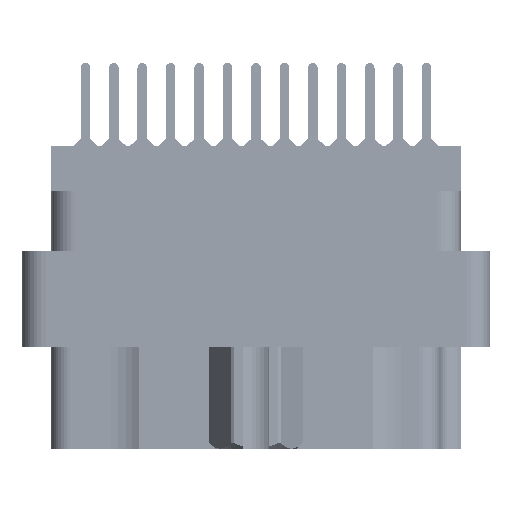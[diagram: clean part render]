
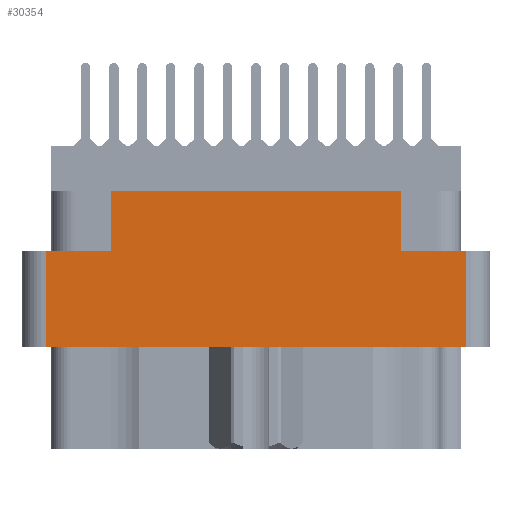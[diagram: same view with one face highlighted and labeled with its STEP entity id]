
A CAD part, left-side view. The second image highlights one B-rep face of the part: STEP entity #30354.
In plain terms, the highlighted planar face has unit normal (-1, 0, 0).
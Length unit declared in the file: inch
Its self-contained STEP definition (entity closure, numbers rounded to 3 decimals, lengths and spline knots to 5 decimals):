
#2329 = DIRECTION ( 'NONE',  ( 0., 1., 0. ) ) ;
#4207 = EDGE_LOOP ( 'NONE', ( #23088, #5940, #24946, #58882, #9343, #20774, #22834, #62159 ) ) ;
#4234 = EDGE_CURVE ( 'NONE', #32977, #33149, #74089, .T. ) ;
#4402 = VECTOR ( 'NONE', #29877, 39.37008 ) ;
#5191 = EDGE_CURVE ( 'NONE', #11066, #46096, #27409, .T. ) ;
#5940 = ORIENTED_EDGE ( 'NONE', *, *, #13438, .T. ) ;
#7363 = CARTESIAN_POINT ( 'NONE',  ( -1.359, 0.555, -0.798 ) ) ;
#7445 = AXIS2_PLACEMENT_3D ( 'NONE', #15939, #22190, #61098 ) ;
#8435 = CARTESIAN_POINT ( 'NONE',  ( -1.359, -0.555, -0.529 ) ) ;
#9343 = ORIENTED_EDGE ( 'NONE', *, *, #72518, .F. ) ;
#11066 = VERTEX_POINT ( 'NONE', #36326 ) ;
#12417 = CARTESIAN_POINT ( 'NONE',  ( -1.359, -0.555, -0.277 ) ) ;
#13404 = CARTESIAN_POINT ( 'NONE',  ( -1.359, 0.3825, -0.277 ) ) ;
#13438 = EDGE_CURVE ( 'NONE', #58204, #33149, #72020, .T. ) ;
#15939 = CARTESIAN_POINT ( 'NONE',  ( -1.359, -0.617, -0.798 ) ) ;
#17860 = DIRECTION ( 'NONE',  ( 0., 0., 1. ) ) ;
#20774 = ORIENTED_EDGE ( 'NONE', *, *, #37668, .T. ) ;
#22190 = DIRECTION ( 'NONE',  ( -1., 0., 0. ) ) ;
#22834 = ORIENTED_EDGE ( 'NONE', *, *, #73538, .F. ) ;
#23088 = ORIENTED_EDGE ( 'NONE', *, *, #38173, .F. ) ;
#23297 = PLANE ( 'NONE',  #7445 ) ;
#24946 = ORIENTED_EDGE ( 'NONE', *, *, #4234, .F. ) ;
#25122 = VERTEX_POINT ( 'NONE', #71787 ) ;
#27409 = LINE ( 'NONE', #13404, #76890 ) ;
#27895 = DIRECTION ( 'NONE',  ( 0., -1., 0. ) ) ;
#29877 = DIRECTION ( 'NONE',  ( 0., -1., 0. ) ) ;
#30354 = ADVANCED_FACE ( 'NONE', ( #48318 ), #23297, .T. ) ;
#30943 = VERTEX_POINT ( 'NONE', #12417 ) ;
#32977 = VERTEX_POINT ( 'NONE', #8435 ) ;
#33024 = CARTESIAN_POINT ( 'NONE',  ( -1.359, 0., -0.277 ) ) ;
#33149 = VERTEX_POINT ( 'NONE', #68557 ) ;
#36326 = CARTESIAN_POINT ( 'NONE',  ( -1.359, 0.3825, -0.277 ) ) ;
#36775 = VECTOR ( 'NONE', #70302, 39.37008 ) ;
#37668 = EDGE_CURVE ( 'NONE', #46288, #25122, #63082, .T. ) ;
#38173 = EDGE_CURVE ( 'NONE', #58204, #11066, #78127, .T. ) ;
#38374 = CARTESIAN_POINT ( 'NONE',  ( -1.359, 0.617, -0.117 ) ) ;
#39466 = CARTESIAN_POINT ( 'NONE',  ( -1.359, 0.555, -0.277 ) ) ;
#39832 = LINE ( 'NONE', #33024, #76165 ) ;
#41041 = CARTESIAN_POINT ( 'NONE',  ( -1.359, 0., -0.529 ) ) ;
#41786 = CARTESIAN_POINT ( 'NONE',  ( -1.359, 0., -0.277 ) ) ;
#46096 = VERTEX_POINT ( 'NONE', #60610 ) ;
#46288 = VERTEX_POINT ( 'NONE', #75838 ) ;
#46964 = DIRECTION ( 'NONE',  ( 0., 0., 1. ) ) ;
#47812 = LINE ( 'NONE', #38374, #36775 ) ;
#48318 = FACE_OUTER_BOUND ( 'NONE', #4207, .T. ) ;
#50732 = VECTOR ( 'NONE', #77898, 39.37008 ) ;
#53866 = VECTOR ( 'NONE', #2329, 39.37008 ) ;
#55731 = LINE ( 'NONE', #73322, #68923 ) ;
#57012 = VECTOR ( 'NONE', #17860, 39.37008 ) ;
#58204 = VERTEX_POINT ( 'NONE', #39466 ) ;
#58272 = EDGE_CURVE ( 'NONE', #32977, #30943, #55731, .T. ) ;
#58882 = ORIENTED_EDGE ( 'NONE', *, *, #58272, .T. ) ;
#60610 = CARTESIAN_POINT ( 'NONE',  ( -1.359, 0.3825, -0.117 ) ) ;
#61098 = DIRECTION ( 'NONE',  ( 0., 0., 1. ) ) ;
#62159 = ORIENTED_EDGE ( 'NONE', *, *, #5191, .F. ) ;
#63082 = LINE ( 'NONE', #68984, #57012 ) ;
#68557 = CARTESIAN_POINT ( 'NONE',  ( -1.359, 0.555, -0.529 ) ) ;
#68923 = VECTOR ( 'NONE', #78933, 39.37008 ) ;
#68984 = CARTESIAN_POINT ( 'NONE',  ( -1.359, -0.3825, -0.277 ) ) ;
#70302 = DIRECTION ( 'NONE',  ( 0., -1., 0. ) ) ;
#71787 = CARTESIAN_POINT ( 'NONE',  ( -1.359, -0.3825, -0.117 ) ) ;
#72020 = LINE ( 'NONE', #7363, #50732 ) ;
#72518 = EDGE_CURVE ( 'NONE', #46288, #30943, #39832, .T. ) ;
#73322 = CARTESIAN_POINT ( 'NONE',  ( -1.359, -0.555, -0.798 ) ) ;
#73538 = EDGE_CURVE ( 'NONE', #46096, #25122, #47812, .T. ) ;
#74089 = LINE ( 'NONE', #41041, #53866 ) ;
#75838 = CARTESIAN_POINT ( 'NONE',  ( -1.359, -0.3825, -0.277 ) ) ;
#76165 = VECTOR ( 'NONE', #27895, 39.37008 ) ;
#76890 = VECTOR ( 'NONE', #46964, 39.37008 ) ;
#77898 = DIRECTION ( 'NONE',  ( 0., 0., -1. ) ) ;
#78127 = LINE ( 'NONE', #41786, #4402 ) ;
#78933 = DIRECTION ( 'NONE',  ( 0., 0., 1. ) ) ;
